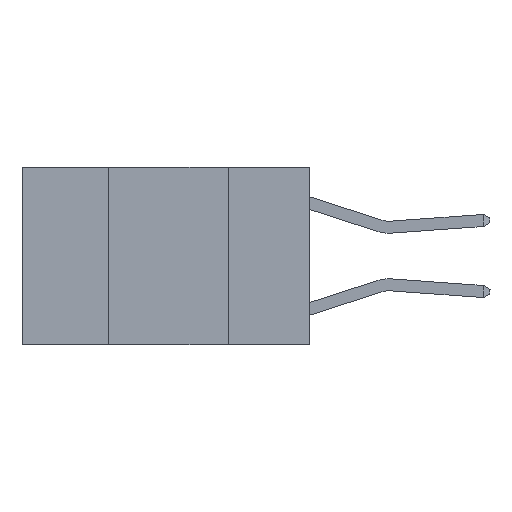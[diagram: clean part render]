
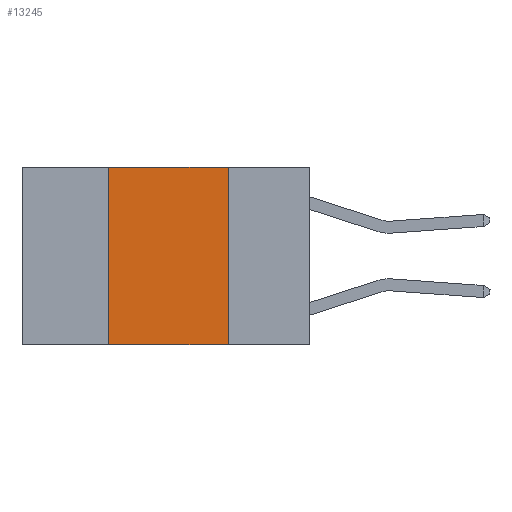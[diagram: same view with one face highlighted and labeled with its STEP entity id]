
A CAD part, left-side view. The second image highlights one B-rep face of the part: STEP entity #13245.
In plain terms, the highlighted planar face has unit normal (-1, 0, 0).
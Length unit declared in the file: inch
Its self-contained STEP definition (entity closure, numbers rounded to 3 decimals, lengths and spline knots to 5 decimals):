
#3807 = LINE ( 'NONE', #20402, #14557 ) ;
#4753 = DIRECTION ( 'NONE',  ( 1., 0., 0. ) ) ;
#4925 = VERTEX_POINT ( 'NONE', #5552 ) ;
#4981 = VECTOR ( 'NONE', #5641, 39.37008 ) ;
#5552 = CARTESIAN_POINT ( 'NONE',  ( 0., 0.42, 0. ) ) ;
#5562 = EDGE_CURVE ( 'NONE', #22273, #23300, #13957, .T. ) ;
#5641 = DIRECTION ( 'NONE',  ( 0., 0., 1. ) ) ;
#6560 = ORIENTED_EDGE ( 'NONE', *, *, #19153, .F. ) ;
#7464 = CARTESIAN_POINT ( 'NONE',  ( 0., 0.6, 0. ) ) ;
#7739 = EDGE_LOOP ( 'NONE', ( #6560, #21669, #24806, #24166 ) ) ;
#9900 = VECTOR ( 'NONE', #16187, 39.37008 ) ;
#10372 = LINE ( 'NONE', #19735, #4981 ) ;
#12133 = AXIS2_PLACEMENT_3D ( 'NONE', #14786, #4753, #18829 ) ;
#13245 = ADVANCED_FACE ( 'NONE', ( #13631 ), #24830, .F. ) ;
#13631 = FACE_OUTER_BOUND ( 'NONE', #7739, .T. ) ;
#13957 = LINE ( 'NONE', #21037, #18660 ) ;
#14325 = DIRECTION ( 'NONE',  ( 0., 0., -1. ) ) ;
#14557 = VECTOR ( 'NONE', #14325, 39.37008 ) ;
#14786 = CARTESIAN_POINT ( 'NONE',  ( 0., 0.6, 0. ) ) ;
#16112 = EDGE_CURVE ( 'NONE', #22273, #4925, #10372, .T. ) ;
#16187 = DIRECTION ( 'NONE',  ( 0., -1., 0. ) ) ;
#16566 = VERTEX_POINT ( 'NONE', #23026 ) ;
#18660 = VECTOR ( 'NONE', #23052, 39.37008 ) ;
#18829 = DIRECTION ( 'NONE',  ( 0., 0., -1. ) ) ;
#19153 = EDGE_CURVE ( 'NONE', #16566, #23300, #3807, .T. ) ;
#19735 = CARTESIAN_POINT ( 'NONE',  ( 0., 0.42, 0. ) ) ;
#20402 = CARTESIAN_POINT ( 'NONE',  ( 0., 0.17, 0. ) ) ;
#20541 = CARTESIAN_POINT ( 'NONE',  ( 0., 0.42, -0.37 ) ) ;
#20595 = LINE ( 'NONE', #7464, #9900 ) ;
#21037 = CARTESIAN_POINT ( 'NONE',  ( 0., 0.6, -0.37 ) ) ;
#21669 = ORIENTED_EDGE ( 'NONE', *, *, #23901, .F. ) ;
#22273 = VERTEX_POINT ( 'NONE', #20541 ) ;
#23026 = CARTESIAN_POINT ( 'NONE',  ( 0., 0.17, 0. ) ) ;
#23052 = DIRECTION ( 'NONE',  ( 0., -1., 0. ) ) ;
#23300 = VERTEX_POINT ( 'NONE', #23308 ) ;
#23308 = CARTESIAN_POINT ( 'NONE',  ( 0., 0.17, -0.37 ) ) ;
#23901 = EDGE_CURVE ( 'NONE', #4925, #16566, #20595, .T. ) ;
#24166 = ORIENTED_EDGE ( 'NONE', *, *, #5562, .T. ) ;
#24806 = ORIENTED_EDGE ( 'NONE', *, *, #16112, .F. ) ;
#24830 = PLANE ( 'NONE',  #12133 ) ;
